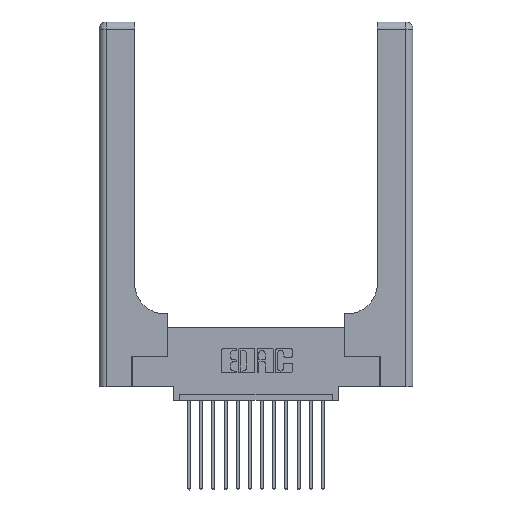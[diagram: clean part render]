
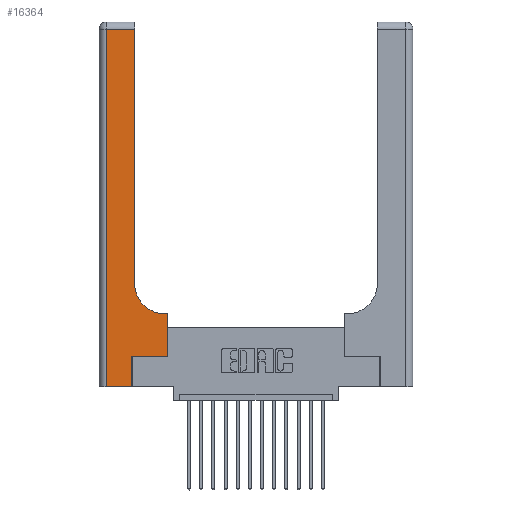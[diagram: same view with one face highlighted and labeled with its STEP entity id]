
A CAD part, top view. The second image highlights one B-rep face of the part: STEP entity #16364.
In plain terms, the highlighted planar face has unit normal (0, 0, 1).
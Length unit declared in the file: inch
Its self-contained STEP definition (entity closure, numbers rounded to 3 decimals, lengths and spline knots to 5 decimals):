
#737 = CARTESIAN_POINT ( 'NONE',  ( 0.5585, 0.25, 0.37 ) ) ;
#818 = EDGE_CURVE ( 'NONE', #14658, #17886, #8943, .T. ) ;
#938 = DIRECTION ( 'NONE',  ( 0., 1., 0. ) ) ;
#991 = EDGE_CURVE ( 'NONE', #17886, #14667, #17801, .T. ) ;
#1133 = ORIENTED_EDGE ( 'NONE', *, *, #10363, .T. ) ;
#1399 = ORIENTED_EDGE ( 'NONE', *, *, #7244, .T. ) ;
#1415 = VERTEX_POINT ( 'NONE', #3562 ) ;
#1486 = LINE ( 'NONE', #12351, #16379 ) ;
#2093 = CARTESIAN_POINT ( 'NONE',  ( 0., 0., 0.37 ) ) ;
#2465 = DIRECTION ( 'NONE',  ( -1., 0., 0. ) ) ;
#3522 = FACE_OUTER_BOUND ( 'NONE', #17103, .T. ) ;
#3562 = CARTESIAN_POINT ( 'NONE',  ( 0.269, 0., 0.37 ) ) ;
#4096 = VECTOR ( 'NONE', #11902, 39.37008 ) ;
#4149 = VECTOR ( 'NONE', #16800, 39.37008 ) ;
#5428 = EDGE_CURVE ( 'NONE', #1415, #10473, #1486, .T. ) ;
#5530 = ORIENTED_EDGE ( 'NONE', *, *, #5428, .T. ) ;
#5735 = CARTESIAN_POINT ( 'NONE',  ( 0.5585, 0.25, 0.37 ) ) ;
#5845 = LINE ( 'NONE', #9590, #12973 ) ;
#6385 = VERTEX_POINT ( 'NONE', #5735 ) ;
#6433 = VERTEX_POINT ( 'NONE', #11295 ) ;
#6594 = LINE ( 'NONE', #11064, #4149 ) ;
#6846 = CARTESIAN_POINT ( 'NONE',  ( 0.269, 0.25, 0.37 ) ) ;
#7117 = DIRECTION ( 'NONE',  ( 0., -1., 0. ) ) ;
#7204 = CARTESIAN_POINT ( 'NONE',  ( 0.5415, 0.6, 0.37 ) ) ;
#7220 = DIRECTION ( 'NONE',  ( 0., 1., 0. ) ) ;
#7244 = EDGE_CURVE ( 'NONE', #14667, #16176, #16303, .T. ) ;
#7483 = LINE ( 'NONE', #10066, #15918 ) ;
#8249 = DIRECTION ( 'NONE',  ( 0., 0., -1. ) ) ;
#8621 = CARTESIAN_POINT ( 'NONE',  ( 0.2915, 0.85, 0.37 ) ) ;
#8734 = VECTOR ( 'NONE', #7220, 39.37008 ) ;
#8943 = CIRCLE ( 'NONE', #14760, 0.25 ) ;
#9036 = LINE ( 'NONE', #737, #12612 ) ;
#9550 = PLANE ( 'NONE',  #11684 ) ;
#9590 = CARTESIAN_POINT ( 'NONE',  ( 0.2915, 0.6, 0.37 ) ) ;
#9880 = ORIENTED_EDGE ( 'NONE', *, *, #10237, .T. ) ;
#10066 = CARTESIAN_POINT ( 'NONE',  ( 0.06, 3., 0.37 ) ) ;
#10198 = EDGE_CURVE ( 'NONE', #10473, #6385, #6594, .T. ) ;
#10237 = EDGE_CURVE ( 'NONE', #16176, #6433, #7483, .T. ) ;
#10310 = ORIENTED_EDGE ( 'NONE', *, *, #991, .T. ) ;
#10363 = EDGE_CURVE ( 'NONE', #6385, #11993, #9036, .T. ) ;
#10473 = VERTEX_POINT ( 'NONE', #6846 ) ;
#10525 = ORIENTED_EDGE ( 'NONE', *, *, #10198, .T. ) ;
#11064 = CARTESIAN_POINT ( 'NONE',  ( 0.269, 0.25, 0.37 ) ) ;
#11165 = CARTESIAN_POINT ( 'NONE',  ( 0.2915, 3., 0.37 ) ) ;
#11295 = CARTESIAN_POINT ( 'NONE',  ( 0.06, 0., 0.37 ) ) ;
#11684 = AXIS2_PLACEMENT_3D ( 'NONE', #16655, #8249, #18133 ) ;
#11825 = CARTESIAN_POINT ( 'NONE',  ( 0.5585, 0.6, 0.37 ) ) ;
#11902 = DIRECTION ( 'NONE',  ( -1., 0., 0. ) ) ;
#11993 = VERTEX_POINT ( 'NONE', #11825 ) ;
#12293 = CARTESIAN_POINT ( 'NONE',  ( 0.06, 2.94, 0.37 ) ) ;
#12294 = DIRECTION ( 'NONE',  ( 0., 0., -1. ) ) ;
#12351 = CARTESIAN_POINT ( 'NONE',  ( 0.269, 0., 0.37 ) ) ;
#12612 = VECTOR ( 'NONE', #938, 39.37008 ) ;
#12890 = DIRECTION ( 'NONE',  ( 0., 1., 0. ) ) ;
#12945 = CARTESIAN_POINT ( 'NONE',  ( 0.2915, 2.94, 0.37 ) ) ;
#12973 = VECTOR ( 'NONE', #2465, 39.37008 ) ;
#13260 = CARTESIAN_POINT ( 'NONE',  ( 0., 2.94, 0.37 ) ) ;
#13578 = VECTOR ( 'NONE', #17666, 39.37008 ) ;
#14483 = ORIENTED_EDGE ( 'NONE', *, *, #17188, .T. ) ;
#14658 = VERTEX_POINT ( 'NONE', #7204 ) ;
#14667 = VERTEX_POINT ( 'NONE', #12945 ) ;
#14760 = AXIS2_PLACEMENT_3D ( 'NONE', #15079, #12294, #15064 ) ;
#14801 = EDGE_CURVE ( 'NONE', #6433, #1415, #15547, .T. ) ;
#15064 = DIRECTION ( 'NONE',  ( 1., 0., 0. ) ) ;
#15079 = CARTESIAN_POINT ( 'NONE',  ( 0.5415, 0.85, 0.37 ) ) ;
#15318 = ORIENTED_EDGE ( 'NONE', *, *, #14801, .T. ) ;
#15480 = ORIENTED_EDGE ( 'NONE', *, *, #818, .T. ) ;
#15547 = LINE ( 'NONE', #2093, #13578 ) ;
#15918 = VECTOR ( 'NONE', #7117, 39.37008 ) ;
#16176 = VERTEX_POINT ( 'NONE', #12293 ) ;
#16303 = LINE ( 'NONE', #13260, #4096 ) ;
#16364 = ADVANCED_FACE ( 'NONE', ( #3522 ), #9550, .F. ) ;
#16379 = VECTOR ( 'NONE', #12890, 39.37008 ) ;
#16655 = CARTESIAN_POINT ( 'NONE',  ( 0., 3., 0.37 ) ) ;
#16800 = DIRECTION ( 'NONE',  ( 1., 0., 0. ) ) ;
#17103 = EDGE_LOOP ( 'NONE', ( #10310, #1399, #9880, #15318, #5530, #10525, #1133, #14483, #15480 ) ) ;
#17188 = EDGE_CURVE ( 'NONE', #11993, #14658, #5845, .T. ) ;
#17666 = DIRECTION ( 'NONE',  ( 1., 0., 0. ) ) ;
#17801 = LINE ( 'NONE', #11165, #8734 ) ;
#17886 = VERTEX_POINT ( 'NONE', #8621 ) ;
#18133 = DIRECTION ( 'NONE',  ( -1., 0., 0. ) ) ;
